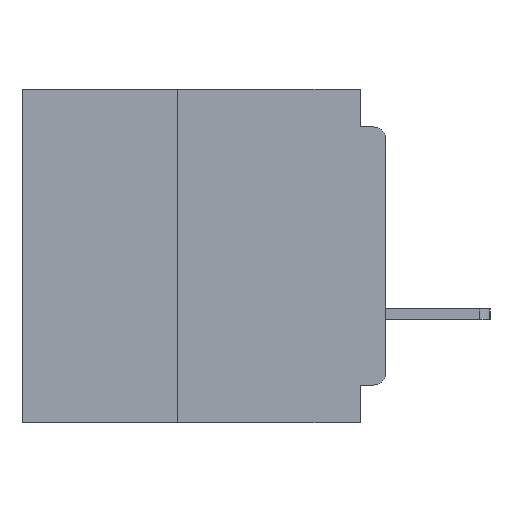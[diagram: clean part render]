
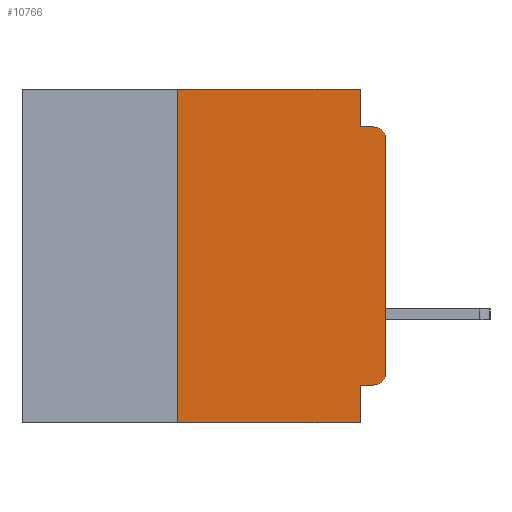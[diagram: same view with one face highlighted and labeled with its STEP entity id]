
A CAD part, left-side view. The second image highlights one B-rep face of the part: STEP entity #10766.
In plain terms, the highlighted planar face has unit normal (-1, 0, 0).
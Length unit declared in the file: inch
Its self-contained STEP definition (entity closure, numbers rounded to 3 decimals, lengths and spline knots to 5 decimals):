
#147 = VECTOR ( 'NONE', #29950, 39.37008 ) ;
#285 = DIRECTION ( 'NONE',  ( 0., 0., -1. ) ) ;
#1430 = LINE ( 'NONE', #30745, #15032 ) ;
#2835 = EDGE_CURVE ( 'NONE', #26335, #15910, #5104, .T. ) ;
#4063 = VECTOR ( 'NONE', #4188, 39.37008 ) ;
#4188 = DIRECTION ( 'NONE',  ( 0., 0., 1. ) ) ;
#4444 = CARTESIAN_POINT ( 'NONE',  ( 0., 0.437, 0. ) ) ;
#4485 = AXIS2_PLACEMENT_3D ( 'NONE', #5009, #24003, #7725 ) ;
#4493 = CARTESIAN_POINT ( 'NONE',  ( 0., 0.031, 0. ) ) ;
#4983 = CIRCLE ( 'NONE', #4485, 0.015 ) ;
#5009 = CARTESIAN_POINT ( 'NONE',  ( 0., 0.015, -0.34 ) ) ;
#5104 = LINE ( 'NONE', #32751, #25950 ) ;
#5317 = LINE ( 'NONE', #22041, #31692 ) ;
#5480 = CARTESIAN_POINT ( 'NONE',  ( 0., 0., 0. ) ) ;
#5860 = CARTESIAN_POINT ( 'NONE',  ( 0., 0.25, -0.4 ) ) ;
#6075 = EDGE_CURVE ( 'NONE', #7454, #29660, #8235, .T. ) ;
#6085 = EDGE_CURVE ( 'NONE', #10521, #13457, #14611, .T. ) ;
#6376 = LINE ( 'NONE', #16325, #32773 ) ;
#6913 = EDGE_CURVE ( 'NONE', #12830, #20237, #1430, .T. ) ;
#6957 = EDGE_CURVE ( 'NONE', #15674, #20669, #14175, .T. ) ;
#7043 = ORIENTED_EDGE ( 'NONE', *, *, #34062, .F. ) ;
#7189 = DIRECTION ( 'NONE',  ( 0., 0., -1. ) ) ;
#7399 = CARTESIAN_POINT ( 'NONE',  ( 0., 0., -0.06 ) ) ;
#7454 = VERTEX_POINT ( 'NONE', #5860 ) ;
#7725 = DIRECTION ( 'NONE',  ( 0., 0., -1. ) ) ;
#8234 = DIRECTION ( 'NONE',  ( 0., 0., -1. ) ) ;
#8235 = LINE ( 'NONE', #29846, #23546 ) ;
#8423 = CARTESIAN_POINT ( 'NONE',  ( 0., 0.031, -0.4 ) ) ;
#9139 = CARTESIAN_POINT ( 'NONE',  ( 0., 0.25, 0. ) ) ;
#9656 = CARTESIAN_POINT ( 'NONE',  ( 0., 0.25, -0.4 ) ) ;
#10490 = EDGE_CURVE ( 'NONE', #13457, #20669, #28958, .T. ) ;
#10521 = VERTEX_POINT ( 'NONE', #27683 ) ;
#10766 = ADVANCED_FACE ( 'NONE', ( #12375 ), #18019, .F. ) ;
#10884 = ORIENTED_EDGE ( 'NONE', *, *, #6957, .F. ) ;
#11007 = EDGE_CURVE ( 'NONE', #15910, #15674, #6376, .T. ) ;
#11379 = CARTESIAN_POINT ( 'NONE',  ( 0., 0.015, -0.06 ) ) ;
#11718 = DIRECTION ( 'NONE',  ( 0., 1., 0. ) ) ;
#11961 = CARTESIAN_POINT ( 'NONE',  ( 0., 0., -0.045 ) ) ;
#12375 = FACE_OUTER_BOUND ( 'NONE', #28341, .T. ) ;
#12830 = VERTEX_POINT ( 'NONE', #13823 ) ;
#13457 = VERTEX_POINT ( 'NONE', #7399 ) ;
#13823 = CARTESIAN_POINT ( 'NONE',  ( 0., 0.015, -0.355 ) ) ;
#14100 = DIRECTION ( 'NONE',  ( 0., 0., -1. ) ) ;
#14175 = LINE ( 'NONE', #11961, #20546 ) ;
#14375 = CARTESIAN_POINT ( 'NONE',  ( 0., 0.031, -0.045 ) ) ;
#14611 = LINE ( 'NONE', #5480, #147 ) ;
#15032 = VECTOR ( 'NONE', #11718, 39.37008 ) ;
#15674 = VERTEX_POINT ( 'NONE', #14375 ) ;
#15910 = VERTEX_POINT ( 'NONE', #4493 ) ;
#16325 = CARTESIAN_POINT ( 'NONE',  ( 0., 0.031, 0. ) ) ;
#17157 = EDGE_CURVE ( 'NONE', #12830, #10521, #4983, .T. ) ;
#18019 = PLANE ( 'NONE',  #34878 ) ;
#19800 = ORIENTED_EDGE ( 'NONE', *, *, #2835, .F. ) ;
#20237 = VERTEX_POINT ( 'NONE', #24840 ) ;
#20546 = VECTOR ( 'NONE', #28249, 39.37008 ) ;
#20669 = VERTEX_POINT ( 'NONE', #23970 ) ;
#21484 = ORIENTED_EDGE ( 'NONE', *, *, #6075, .T. ) ;
#22041 = CARTESIAN_POINT ( 'NONE',  ( 0., 0.031, -0.4 ) ) ;
#22511 = EDGE_CURVE ( 'NONE', #20237, #29660, #5317, .T. ) ;
#23463 = DIRECTION ( 'NONE',  ( 1., 0., 0. ) ) ;
#23546 = VECTOR ( 'NONE', #24466, 39.37008 ) ;
#23970 = CARTESIAN_POINT ( 'NONE',  ( 0., 0.015, -0.045 ) ) ;
#24003 = DIRECTION ( 'NONE',  ( -1., 0., 0. ) ) ;
#24045 = ORIENTED_EDGE ( 'NONE', *, *, #22511, .F. ) ;
#24466 = DIRECTION ( 'NONE',  ( 0., -1., 0. ) ) ;
#24840 = CARTESIAN_POINT ( 'NONE',  ( 0., 0.031, -0.355 ) ) ;
#25747 = LINE ( 'NONE', #9656, #4063 ) ;
#25950 = VECTOR ( 'NONE', #32718, 39.37008 ) ;
#26211 = ORIENTED_EDGE ( 'NONE', *, *, #11007, .F. ) ;
#26335 = VERTEX_POINT ( 'NONE', #9139 ) ;
#26646 = ORIENTED_EDGE ( 'NONE', *, *, #17157, .T. ) ;
#27683 = CARTESIAN_POINT ( 'NONE',  ( 0., 0., -0.34 ) ) ;
#28249 = DIRECTION ( 'NONE',  ( 0., -1., 0. ) ) ;
#28341 = EDGE_LOOP ( 'NONE', ( #30869, #31719, #10884, #26211, #19800, #7043, #21484, #24045, #33038, #26646 ) ) ;
#28958 = CIRCLE ( 'NONE', #31911, 0.015 ) ;
#29660 = VERTEX_POINT ( 'NONE', #8423 ) ;
#29846 = CARTESIAN_POINT ( 'NONE',  ( 0., 0.437, -0.4 ) ) ;
#29950 = DIRECTION ( 'NONE',  ( 0., 0., 1. ) ) ;
#30397 = DIRECTION ( 'NONE',  ( -1., 0., 0. ) ) ;
#30745 = CARTESIAN_POINT ( 'NONE',  ( 0., 0., -0.355 ) ) ;
#30869 = ORIENTED_EDGE ( 'NONE', *, *, #6085, .T. ) ;
#31692 = VECTOR ( 'NONE', #285, 39.37008 ) ;
#31719 = ORIENTED_EDGE ( 'NONE', *, *, #10490, .T. ) ;
#31911 = AXIS2_PLACEMENT_3D ( 'NONE', #11379, #30397, #14100 ) ;
#32718 = DIRECTION ( 'NONE',  ( 0., -1., 0. ) ) ;
#32751 = CARTESIAN_POINT ( 'NONE',  ( 0., 0.437, 0. ) ) ;
#32773 = VECTOR ( 'NONE', #8234, 39.37008 ) ;
#33038 = ORIENTED_EDGE ( 'NONE', *, *, #6913, .F. ) ;
#34062 = EDGE_CURVE ( 'NONE', #7454, #26335, #25747, .T. ) ;
#34878 = AXIS2_PLACEMENT_3D ( 'NONE', #4444, #23463, #7189 ) ;
